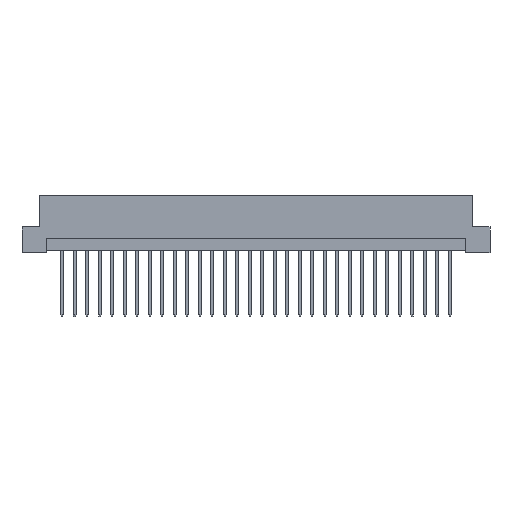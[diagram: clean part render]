
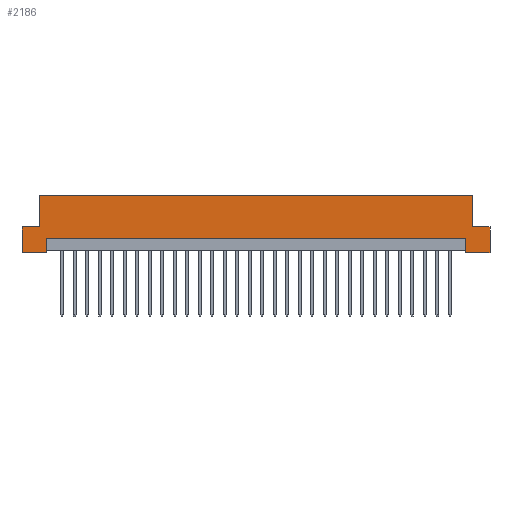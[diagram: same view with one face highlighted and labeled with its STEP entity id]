
A CAD part, front view. The second image highlights one B-rep face of the part: STEP entity #2186.
In plain terms, the highlighted planar face has unit normal (0, -1, 0).
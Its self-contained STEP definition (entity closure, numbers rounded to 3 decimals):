
#134 = DIRECTION ( 'NONE',  ( 1., 0., 0. ) ) ;
#179 = CARTESIAN_POINT ( 'NONE',  ( -47.5, 0., 0. ) ) ;
#572 = CARTESIAN_POINT ( 'NONE',  ( 44., 0., 5.2 ) ) ;
#767 = LINE ( 'NONE', #6140, #16775 ) ;
#874 = DIRECTION ( 'NONE',  ( 0., 0., -1. ) ) ;
#941 = DIRECTION ( 'NONE',  ( 1., 0., 0. ) ) ;
#1184 = EDGE_CURVE ( 'NONE', #5834, #4192, #14687, .T. ) ;
#1257 = CARTESIAN_POINT ( 'NONE',  ( 47.5, 0., 0. ) ) ;
#1424 = DIRECTION ( 'NONE',  ( 0., 0., 1. ) ) ;
#1746 = EDGE_CURVE ( 'NONE', #12444, #6362, #5586, .T. ) ;
#1847 = VERTEX_POINT ( 'NONE', #5768 ) ;
#1941 = DIRECTION ( 'NONE',  ( 0., 1., 0. ) ) ;
#2049 = VECTOR ( 'NONE', #12318, 1000. ) ;
#2117 = CARTESIAN_POINT ( 'NONE',  ( 47.5, 0., 0. ) ) ;
#2186 = ADVANCED_FACE ( 'NONE', ( #16160 ), #4489, .F. ) ;
#2679 = EDGE_CURVE ( 'NONE', #7567, #6362, #7008, .T. ) ;
#2694 = EDGE_CURVE ( 'NONE', #1847, #15216, #4556, .T. ) ;
#3122 = CARTESIAN_POINT ( 'NONE',  ( 42.6, 0., 0.5 ) ) ;
#3811 = CARTESIAN_POINT ( 'NONE',  ( -42.6, 0., 2.9 ) ) ;
#3824 = CARTESIAN_POINT ( 'NONE',  ( 42.6, 0., 2.9 ) ) ;
#4110 = VECTOR ( 'NONE', #17137, 1000. ) ;
#4192 = VERTEX_POINT ( 'NONE', #4460 ) ;
#4193 = CARTESIAN_POINT ( 'NONE',  ( 44., 0., 5.2 ) ) ;
#4460 = CARTESIAN_POINT ( 'NONE',  ( -47.5, 0., 0. ) ) ;
#4489 = PLANE ( 'NONE',  #8102 ) ;
#4556 = LINE ( 'NONE', #12396, #16599 ) ;
#4895 = VECTOR ( 'NONE', #874, 1000. ) ;
#5298 = ORIENTED_EDGE ( 'NONE', *, *, #16102, .T. ) ;
#5383 = DIRECTION ( 'NONE',  ( 0., 0., 1. ) ) ;
#5516 = CARTESIAN_POINT ( 'NONE',  ( 44., 0., 11.6 ) ) ;
#5586 = LINE ( 'NONE', #3122, #14865 ) ;
#5644 = ORIENTED_EDGE ( 'NONE', *, *, #8836, .F. ) ;
#5768 = CARTESIAN_POINT ( 'NONE',  ( -47.5, 0., 5.2 ) ) ;
#5834 = VERTEX_POINT ( 'NONE', #17149 ) ;
#6140 = CARTESIAN_POINT ( 'NONE',  ( 47.5, 0., 5.2 ) ) ;
#6362 = VERTEX_POINT ( 'NONE', #14643 ) ;
#6411 = CARTESIAN_POINT ( 'NONE',  ( -47.5, 0., 0. ) ) ;
#6423 = VERTEX_POINT ( 'NONE', #13764 ) ;
#6454 = LINE ( 'NONE', #3824, #4110 ) ;
#6504 = EDGE_LOOP ( 'NONE', ( #12055, #17120, #15956, #11415, #15337, #5298, #7371, #5644, #12670, #13843, #10048, #15307 ) ) ;
#6711 = VECTOR ( 'NONE', #11245, 1000. ) ;
#6985 = DIRECTION ( 'NONE',  ( 0., 0., -1. ) ) ;
#7008 = LINE ( 'NONE', #12577, #6711 ) ;
#7371 = ORIENTED_EDGE ( 'NONE', *, *, #13630, .F. ) ;
#7567 = VERTEX_POINT ( 'NONE', #1257 ) ;
#7872 = LINE ( 'NONE', #8048, #12436 ) ;
#8048 = CARTESIAN_POINT ( 'NONE',  ( -47.5, 0., 11.6 ) ) ;
#8102 = AXIS2_PLACEMENT_3D ( 'NONE', #16498, #1941, #5383 ) ;
#8245 = EDGE_CURVE ( 'NONE', #12030, #7567, #9068, .T. ) ;
#8792 = DIRECTION ( 'NONE',  ( 0., 0., 1. ) ) ;
#8836 = EDGE_CURVE ( 'NONE', #15216, #6423, #9356, .T. ) ;
#9068 = LINE ( 'NONE', #2117, #4895 ) ;
#9356 = LINE ( 'NONE', #16251, #12508 ) ;
#9657 = LINE ( 'NONE', #4193, #13908 ) ;
#10048 = ORIENTED_EDGE ( 'NONE', *, *, #1184, .F. ) ;
#10187 = EDGE_CURVE ( 'NONE', #11851, #12030, #767, .T. ) ;
#10642 = CARTESIAN_POINT ( 'NONE',  ( -42.6, 0., 0.5 ) ) ;
#10751 = EDGE_CURVE ( 'NONE', #12444, #15643, #6454, .T. ) ;
#11245 = DIRECTION ( 'NONE',  ( -1., 0., 0. ) ) ;
#11415 = ORIENTED_EDGE ( 'NONE', *, *, #8245, .F. ) ;
#11473 = CARTESIAN_POINT ( 'NONE',  ( 42.6, 0., 2.9 ) ) ;
#11851 = VERTEX_POINT ( 'NONE', #572 ) ;
#12030 = VERTEX_POINT ( 'NONE', #12831 ) ;
#12055 = ORIENTED_EDGE ( 'NONE', *, *, #10751, .F. ) ;
#12250 = LINE ( 'NONE', #179, #16728 ) ;
#12318 = DIRECTION ( 'NONE',  ( 0., 0., -1. ) ) ;
#12396 = CARTESIAN_POINT ( 'NONE',  ( -47.5, 0., 5.2 ) ) ;
#12436 = VECTOR ( 'NONE', #134, 1000. ) ;
#12444 = VERTEX_POINT ( 'NONE', #11473 ) ;
#12508 = VECTOR ( 'NONE', #1424, 1000. ) ;
#12577 = CARTESIAN_POINT ( 'NONE',  ( -47.5, 0., 0. ) ) ;
#12670 = ORIENTED_EDGE ( 'NONE', *, *, #2694, .F. ) ;
#12831 = CARTESIAN_POINT ( 'NONE',  ( 47.5, 0., 5.2 ) ) ;
#13460 = VECTOR ( 'NONE', #16114, 1000. ) ;
#13630 = EDGE_CURVE ( 'NONE', #6423, #17163, #7872, .T. ) ;
#13764 = CARTESIAN_POINT ( 'NONE',  ( -44., 0., 11.6 ) ) ;
#13812 = DIRECTION ( 'NONE',  ( 1., 0., 0. ) ) ;
#13843 = ORIENTED_EDGE ( 'NONE', *, *, #15851, .F. ) ;
#13908 = VECTOR ( 'NONE', #16020, 1000. ) ;
#14301 = EDGE_CURVE ( 'NONE', #15643, #5834, #14962, .T. ) ;
#14643 = CARTESIAN_POINT ( 'NONE',  ( 42.6, 0., 0. ) ) ;
#14687 = LINE ( 'NONE', #6411, #13460 ) ;
#14865 = VECTOR ( 'NONE', #6985, 1000. ) ;
#14919 = CARTESIAN_POINT ( 'NONE',  ( -44., 0., 5.2 ) ) ;
#14962 = LINE ( 'NONE', #10642, #2049 ) ;
#15216 = VERTEX_POINT ( 'NONE', #14919 ) ;
#15307 = ORIENTED_EDGE ( 'NONE', *, *, #14301, .F. ) ;
#15337 = ORIENTED_EDGE ( 'NONE', *, *, #10187, .F. ) ;
#15643 = VERTEX_POINT ( 'NONE', #3811 ) ;
#15851 = EDGE_CURVE ( 'NONE', #4192, #1847, #12250, .T. ) ;
#15956 = ORIENTED_EDGE ( 'NONE', *, *, #2679, .F. ) ;
#16020 = DIRECTION ( 'NONE',  ( 0., 0., 1. ) ) ;
#16102 = EDGE_CURVE ( 'NONE', #11851, #17163, #9657, .T. ) ;
#16114 = DIRECTION ( 'NONE',  ( -1., 0., 0. ) ) ;
#16160 = FACE_OUTER_BOUND ( 'NONE', #6504, .T. ) ;
#16251 = CARTESIAN_POINT ( 'NONE',  ( -44., 0., 5.2 ) ) ;
#16498 = CARTESIAN_POINT ( 'NONE',  ( -47.5, 0., 11.6 ) ) ;
#16599 = VECTOR ( 'NONE', #13812, 1000. ) ;
#16728 = VECTOR ( 'NONE', #8792, 1000. ) ;
#16775 = VECTOR ( 'NONE', #941, 1000. ) ;
#17120 = ORIENTED_EDGE ( 'NONE', *, *, #1746, .T. ) ;
#17137 = DIRECTION ( 'NONE',  ( -1., 0., 0. ) ) ;
#17149 = CARTESIAN_POINT ( 'NONE',  ( -42.6, 0., 0. ) ) ;
#17163 = VERTEX_POINT ( 'NONE', #5516 ) ;
